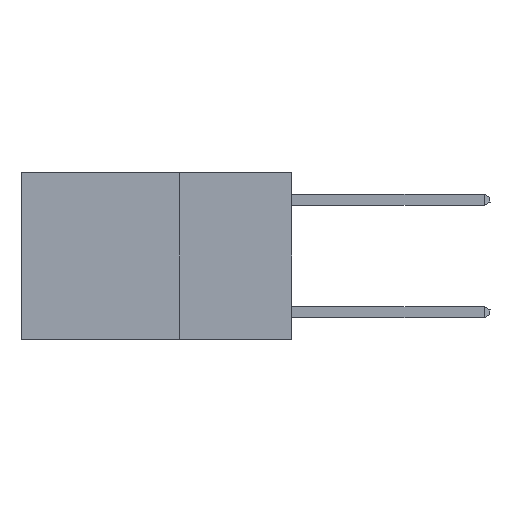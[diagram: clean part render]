
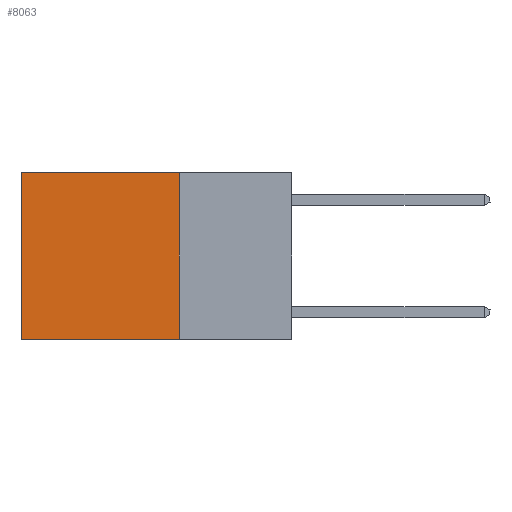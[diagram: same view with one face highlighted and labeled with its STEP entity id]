
A CAD part, left-side view. The second image highlights one B-rep face of the part: STEP entity #8063.
In plain terms, the highlighted planar face has unit normal (-1, 0, 0).
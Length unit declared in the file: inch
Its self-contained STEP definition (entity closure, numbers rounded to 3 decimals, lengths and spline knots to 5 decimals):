
#813 = EDGE_LOOP ( 'NONE', ( #6708, #3754, #7907, #14850 ) ) ;
#1118 = CARTESIAN_POINT ( 'NONE',  ( 0.2625, 0.6, 0. ) ) ;
#1172 = CARTESIAN_POINT ( 'NONE',  ( 0.2625, 0.6, -0.37 ) ) ;
#1300 = VERTEX_POINT ( 'NONE', #19066 ) ;
#2559 = VECTOR ( 'NONE', #8845, 39.37008 ) ;
#3126 = FACE_OUTER_BOUND ( 'NONE', #813, .T. ) ;
#3754 = ORIENTED_EDGE ( 'NONE', *, *, #29411, .F. ) ;
#3787 = CARTESIAN_POINT ( 'NONE',  ( 0.2625, 0.25, 0. ) ) ;
#6708 = ORIENTED_EDGE ( 'NONE', *, *, #16034, .T. ) ;
#7700 = DIRECTION ( 'NONE',  ( 0., 1., 0. ) ) ;
#7907 = ORIENTED_EDGE ( 'NONE', *, *, #19570, .F. ) ;
#7957 = LINE ( 'NONE', #1118, #15779 ) ;
#8063 = ADVANCED_FACE ( 'NONE', ( #3126 ), #14664, .F. ) ;
#8845 = DIRECTION ( 'NONE',  ( 0., 1., 0. ) ) ;
#9704 = AXIS2_PLACEMENT_3D ( 'NONE', #26655, #28473, #12691 ) ;
#11628 = VECTOR ( 'NONE', #7700, 39.37008 ) ;
#12114 = CARTESIAN_POINT ( 'NONE',  ( 0.2625, 0.25, 0. ) ) ;
#12500 = DIRECTION ( 'NONE',  ( 0., 0., -1. ) ) ;
#12691 = DIRECTION ( 'NONE',  ( 0., 0., -1. ) ) ;
#12706 = LINE ( 'NONE', #12114, #11628 ) ;
#13832 = VERTEX_POINT ( 'NONE', #17815 ) ;
#13993 = VECTOR ( 'NONE', #22846, 39.37008 ) ;
#14664 = PLANE ( 'NONE',  #9704 ) ;
#14850 = ORIENTED_EDGE ( 'NONE', *, *, #25524, .T. ) ;
#15779 = VECTOR ( 'NONE', #12500, 39.37008 ) ;
#16015 = CARTESIAN_POINT ( 'NONE',  ( 0.2625, 0.25, 0. ) ) ;
#16034 = EDGE_CURVE ( 'NONE', #1300, #25652, #7957, .T. ) ;
#16983 = VERTEX_POINT ( 'NONE', #3787 ) ;
#17815 = CARTESIAN_POINT ( 'NONE',  ( 0.2625, 0.25, -0.37 ) ) ;
#18139 = LINE ( 'NONE', #16015, #13993 ) ;
#19066 = CARTESIAN_POINT ( 'NONE',  ( 0.2625, 0.6, 0. ) ) ;
#19570 = EDGE_CURVE ( 'NONE', #16983, #13832, #18139, .T. ) ;
#22846 = DIRECTION ( 'NONE',  ( 0., 0., -1. ) ) ;
#24949 = CARTESIAN_POINT ( 'NONE',  ( 0.2625, 0.25, -0.37 ) ) ;
#25524 = EDGE_CURVE ( 'NONE', #16983, #1300, #12706, .T. ) ;
#25652 = VERTEX_POINT ( 'NONE', #1172 ) ;
#26655 = CARTESIAN_POINT ( 'NONE',  ( 0.2625, 0.25, 0. ) ) ;
#27195 = LINE ( 'NONE', #24949, #2559 ) ;
#28473 = DIRECTION ( 'NONE',  ( 1., 0., 0. ) ) ;
#29411 = EDGE_CURVE ( 'NONE', #13832, #25652, #27195, .T. ) ;
